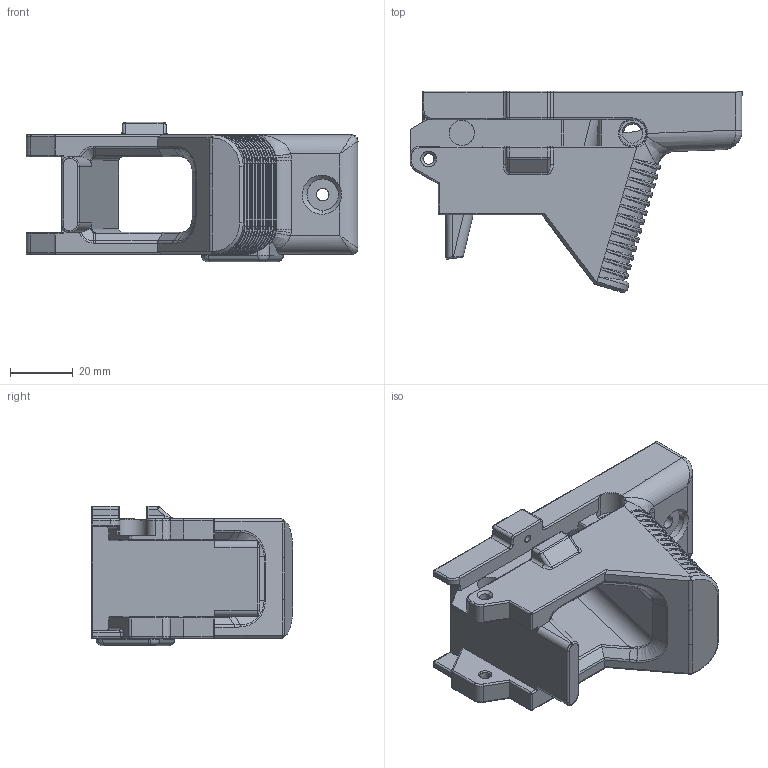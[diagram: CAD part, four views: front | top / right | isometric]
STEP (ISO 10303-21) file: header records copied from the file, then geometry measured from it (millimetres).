
FILE_DESCRIPTION (( 'STEP AP203' ), '1' );
FILE_NAME ('MOD9_V3_Magwell.STEP', '2020-12-23T18:59:59', ( '' ), ( '' ), 'SwSTEP 2.0', 'SolidWorks 2019', '' );
FILE_SCHEMA (( 'CONFIG_CONTROL_DESIGN' ));
Length unit declared in the file: millimetre
Products named in the file (1): MOD9_V3_Magwell
Bounding box: 105.51 x 64.04 x 44.27 mm (x, y, z)
Surface area: 26281.6 mm2 (no closed solid volume)
Topology: 0 solids, 1 shells, 578 faces, 1446 edges, 852 vertices
Faces by surface type: cylinder 234, bspline 158, plane 147, cone 26, torus 13
Entity records: 30446 total; most frequent: CARTESIAN_POINT 18437, ORIENTED_EDGE 2849, DIRECTION 1901, EDGE_CURVE 1426, VERTEX_POINT 852, AXIS2_PLACEMENT_3D 668, B_SPLINE_CURVE_WITH_KNOTS 603, EDGE_LOOP 595
